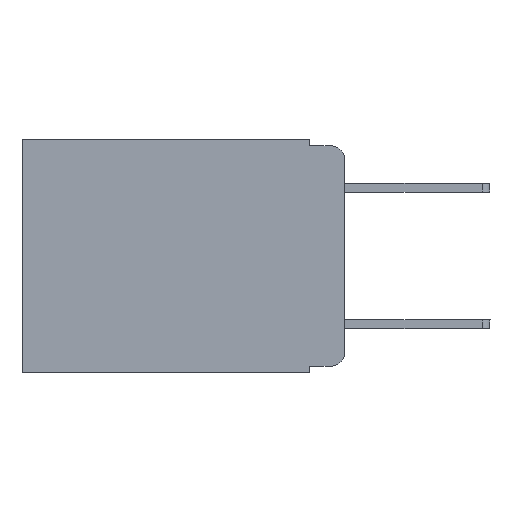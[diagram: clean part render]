
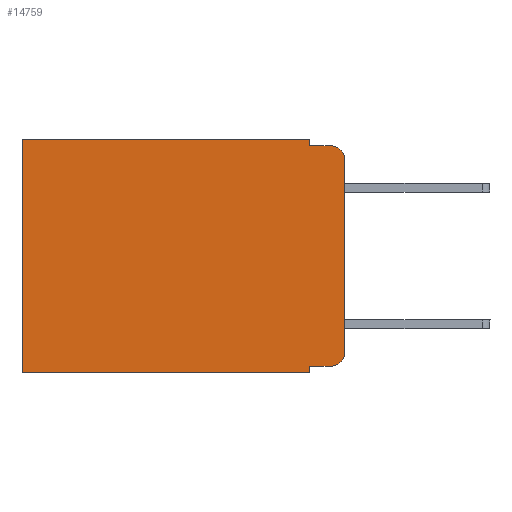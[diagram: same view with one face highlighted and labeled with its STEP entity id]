
A CAD part, left-side view. The second image highlights one B-rep face of the part: STEP entity #14759.
In plain terms, the highlighted planar face has unit normal (-1, 0, 0).
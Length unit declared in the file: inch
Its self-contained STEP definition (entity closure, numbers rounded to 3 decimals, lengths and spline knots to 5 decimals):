
#419 = LINE ( 'NONE', #4522, #17868 ) ;
#424 = LINE ( 'NONE', #17951, #14223 ) ;
#1059 = LINE ( 'NONE', #14748, #8094 ) ;
#1292 = EDGE_CURVE ( 'NONE', #18039, #11955, #1059, .T. ) ;
#1849 = CARTESIAN_POINT ( 'NONE',  ( 0.298, 0.051, -0.01 ) ) ;
#2123 = DIRECTION ( 'NONE',  ( -1., 0., 0. ) ) ;
#2345 = EDGE_CURVE ( 'NONE', #22996, #4590, #19602, .T. ) ;
#2472 = LINE ( 'NONE', #1849, #9766 ) ;
#2758 = CARTESIAN_POINT ( 'NONE',  ( 0.298, 0., 0. ) ) ;
#3318 = EDGE_CURVE ( 'NONE', #4857, #18039, #19559, .T. ) ;
#3549 = VECTOR ( 'NONE', #11518, 39.37008 ) ;
#3759 = CARTESIAN_POINT ( 'NONE',  ( 0.298, 0.051, -0.333 ) ) ;
#3998 = DIRECTION ( 'NONE',  ( 0., 1., 0. ) ) ;
#4376 = ORIENTED_EDGE ( 'NONE', *, *, #14225, .F. ) ;
#4456 = CARTESIAN_POINT ( 'NONE',  ( 0.298, 0.02, -0.01 ) ) ;
#4522 = CARTESIAN_POINT ( 'NONE',  ( 0.298, 0.473, 0. ) ) ;
#4590 = VERTEX_POINT ( 'NONE', #20269 ) ;
#4857 = VERTEX_POINT ( 'NONE', #6664 ) ;
#6208 = DIRECTION ( 'NONE',  ( 1., 0., 0. ) ) ;
#6607 = VERTEX_POINT ( 'NONE', #11398 ) ;
#6664 = CARTESIAN_POINT ( 'NONE',  ( 0.298, 0.051, -0.333 ) ) ;
#7753 = CARTESIAN_POINT ( 'NONE',  ( 0.298, 0.051, 0. ) ) ;
#7867 = ORIENTED_EDGE ( 'NONE', *, *, #7955, .F. ) ;
#7955 = EDGE_CURVE ( 'NONE', #14358, #13655, #424, .T. ) ;
#8094 = VECTOR ( 'NONE', #18590, 39.37008 ) ;
#8308 = LINE ( 'NONE', #3759, #3549 ) ;
#8375 = CARTESIAN_POINT ( 'NONE',  ( 0.298, 0.02, -0.333 ) ) ;
#8733 = ORIENTED_EDGE ( 'NONE', *, *, #3318, .F. ) ;
#9264 = AXIS2_PLACEMENT_3D ( 'NONE', #11230, #2123, #21744 ) ;
#9699 = DIRECTION ( 'NONE',  ( 0., 0., -1. ) ) ;
#9766 = VECTOR ( 'NONE', #16272, 39.37008 ) ;
#9794 = DIRECTION ( 'NONE',  ( -1., 0., 0. ) ) ;
#9807 = CARTESIAN_POINT ( 'NONE',  ( 0.298, 0.473, 0. ) ) ;
#9980 = DIRECTION ( 'NONE',  ( 0., 0., -1. ) ) ;
#10097 = DIRECTION ( 'NONE',  ( 0., 0., -1. ) ) ;
#10103 = CARTESIAN_POINT ( 'NONE',  ( 0.298, 0.051, -0.343 ) ) ;
#10611 = AXIS2_PLACEMENT_3D ( 'NONE', #2758, #6208, #9980 ) ;
#11230 = CARTESIAN_POINT ( 'NONE',  ( 0.298, 0.02, -0.03 ) ) ;
#11398 = CARTESIAN_POINT ( 'NONE',  ( 0.298, 0., -0.03 ) ) ;
#11518 = DIRECTION ( 'NONE',  ( 0., -1., 0. ) ) ;
#11685 = DIRECTION ( 'NONE',  ( 0., 0., -1. ) ) ;
#11955 = VERTEX_POINT ( 'NONE', #16469 ) ;
#12267 = AXIS2_PLACEMENT_3D ( 'NONE', #22094, #9794, #11685 ) ;
#13081 = CARTESIAN_POINT ( 'NONE',  ( 0.298, 0., 0. ) ) ;
#13655 = VERTEX_POINT ( 'NONE', #22161 ) ;
#14223 = VECTOR ( 'NONE', #16284, 39.37008 ) ;
#14225 = EDGE_CURVE ( 'NONE', #13655, #19051, #2472, .T. ) ;
#14358 = VERTEX_POINT ( 'NONE', #7753 ) ;
#14515 = ORIENTED_EDGE ( 'NONE', *, *, #20641, .F. ) ;
#14748 = CARTESIAN_POINT ( 'NONE',  ( 0.298, 0., -0.343 ) ) ;
#14759 = ADVANCED_FACE ( 'NONE', ( #22394 ), #20637, .F. ) ;
#15623 = EDGE_CURVE ( 'NONE', #14358, #17225, #20344, .T. ) ;
#15824 = EDGE_CURVE ( 'NONE', #4857, #22996, #8308, .T. ) ;
#16236 = CARTESIAN_POINT ( 'NONE',  ( 0.298, 0., 0. ) ) ;
#16272 = DIRECTION ( 'NONE',  ( 0., -1., 0. ) ) ;
#16284 = DIRECTION ( 'NONE',  ( 0., 0., -1. ) ) ;
#16327 = ORIENTED_EDGE ( 'NONE', *, *, #15824, .T. ) ;
#16469 = CARTESIAN_POINT ( 'NONE',  ( 0.298, 0.473, -0.343 ) ) ;
#16533 = DIRECTION ( 'NONE',  ( 0., 0., -1. ) ) ;
#17151 = EDGE_CURVE ( 'NONE', #6607, #19051, #18459, .T. ) ;
#17156 = CARTESIAN_POINT ( 'NONE',  ( 0.298, 0.051, 0. ) ) ;
#17225 = VERTEX_POINT ( 'NONE', #9807 ) ;
#17853 = VECTOR ( 'NONE', #10097, 39.37008 ) ;
#17868 = VECTOR ( 'NONE', #9699, 39.37008 ) ;
#17951 = CARTESIAN_POINT ( 'NONE',  ( 0.298, 0.051, 0. ) ) ;
#17992 = EDGE_CURVE ( 'NONE', #17225, #11955, #419, .T. ) ;
#18016 = ORIENTED_EDGE ( 'NONE', *, *, #2345, .T. ) ;
#18039 = VERTEX_POINT ( 'NONE', #10103 ) ;
#18459 = CIRCLE ( 'NONE', #9264, 0.02 ) ;
#18590 = DIRECTION ( 'NONE',  ( 0., 1., 0. ) ) ;
#18853 = ORIENTED_EDGE ( 'NONE', *, *, #17992, .T. ) ;
#19051 = VERTEX_POINT ( 'NONE', #4456 ) ;
#19433 = EDGE_LOOP ( 'NONE', ( #14515, #20309, #4376, #7867, #21885, #18853, #20651, #8733, #16327, #18016 ) ) ;
#19559 = LINE ( 'NONE', #17156, #17853 ) ;
#19602 = CIRCLE ( 'NONE', #12267, 0.02 ) ;
#19746 = VECTOR ( 'NONE', #16533, 39.37008 ) ;
#20269 = CARTESIAN_POINT ( 'NONE',  ( 0.298, 0., -0.313 ) ) ;
#20309 = ORIENTED_EDGE ( 'NONE', *, *, #17151, .T. ) ;
#20344 = LINE ( 'NONE', #13081, #22900 ) ;
#20637 = PLANE ( 'NONE',  #10611 ) ;
#20641 = EDGE_CURVE ( 'NONE', #6607, #4590, #21694, .T. ) ;
#20651 = ORIENTED_EDGE ( 'NONE', *, *, #1292, .F. ) ;
#21694 = LINE ( 'NONE', #16236, #19746 ) ;
#21744 = DIRECTION ( 'NONE',  ( 0., 0., -1. ) ) ;
#21885 = ORIENTED_EDGE ( 'NONE', *, *, #15623, .T. ) ;
#22094 = CARTESIAN_POINT ( 'NONE',  ( 0.298, 0.02, -0.313 ) ) ;
#22161 = CARTESIAN_POINT ( 'NONE',  ( 0.298, 0.051, -0.01 ) ) ;
#22394 = FACE_OUTER_BOUND ( 'NONE', #19433, .T. ) ;
#22900 = VECTOR ( 'NONE', #3998, 39.37008 ) ;
#22996 = VERTEX_POINT ( 'NONE', #8375 ) ;
